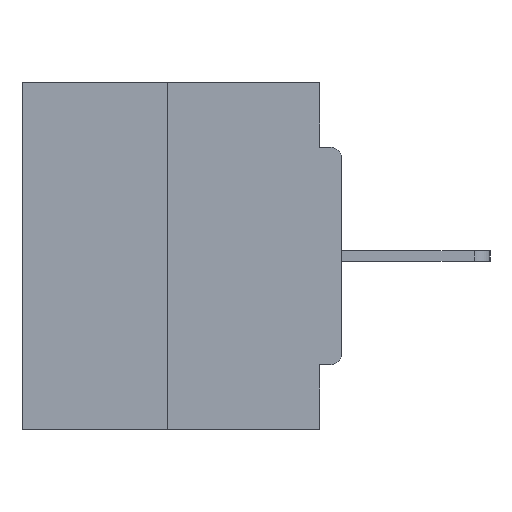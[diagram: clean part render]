
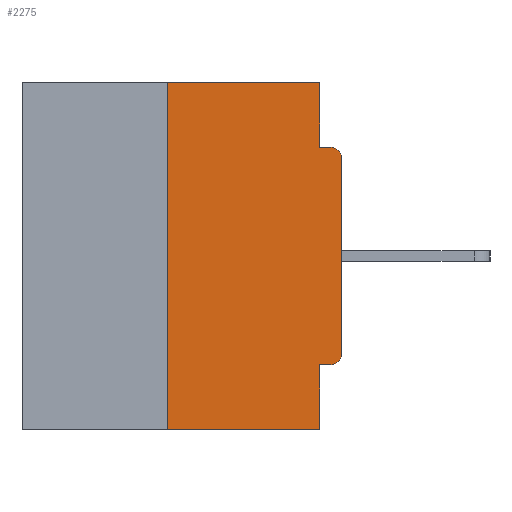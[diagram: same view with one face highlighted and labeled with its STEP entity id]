
A CAD part, left-side view. The second image highlights one B-rep face of the part: STEP entity #2275.
In plain terms, the highlighted planar face has unit normal (-1, 0, 0).
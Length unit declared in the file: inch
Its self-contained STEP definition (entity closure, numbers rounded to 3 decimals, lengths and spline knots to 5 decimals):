
#104 = VECTOR ( 'NONE', #35203, 39.37008 ) ;
#151 = DIRECTION ( 'NONE',  ( 0., 0., -1. ) ) ;
#717 = CARTESIAN_POINT ( 'NONE',  ( 0., 0.031, -0.5 ) ) ;
#1265 = VECTOR ( 'NONE', #12750, 39.37008 ) ;
#1511 = VECTOR ( 'NONE', #16951, 39.37008 ) ;
#1532 = CIRCLE ( 'NONE', #19184, 0.015 ) ;
#1809 = EDGE_CURVE ( 'NONE', #23077, #18736, #36582, .T. ) ;
#2156 = EDGE_CURVE ( 'NONE', #33586, #13961, #5020, .T. ) ;
#2213 = VERTEX_POINT ( 'NONE', #11790 ) ;
#2275 = ADVANCED_FACE ( 'NONE', ( #6070 ), #9224, .F. ) ;
#2962 = DIRECTION ( 'NONE',  ( 0., -1., 0. ) ) ;
#3722 = CARTESIAN_POINT ( 'NONE',  ( 0., 0.015, -0.1085 ) ) ;
#4447 = CARTESIAN_POINT ( 'NONE',  ( 0., 0.031, -0.0935 ) ) ;
#4736 = AXIS2_PLACEMENT_3D ( 'NONE', #36538, #33577, #151 ) ;
#5020 = CIRCLE ( 'NONE', #6319, 0.015 ) ;
#5536 = EDGE_CURVE ( 'NONE', #30319, #26756, #10783, .T. ) ;
#5857 = EDGE_CURVE ( 'NONE', #2213, #18736, #27790, .T. ) ;
#6070 = FACE_OUTER_BOUND ( 'NONE', #24114, .T. ) ;
#6159 = ORIENTED_EDGE ( 'NONE', *, *, #27015, .F. ) ;
#6319 = AXIS2_PLACEMENT_3D ( 'NONE', #11196, #11395, #8246 ) ;
#6888 = EDGE_CURVE ( 'NONE', #33586, #2213, #14207, .T. ) ;
#7771 = ORIENTED_EDGE ( 'NONE', *, *, #5536, .F. ) ;
#8246 = DIRECTION ( 'NONE',  ( 0., 0., -1. ) ) ;
#9224 = PLANE ( 'NONE',  #4736 ) ;
#9358 = CARTESIAN_POINT ( 'NONE',  ( 0., 0.25, 0. ) ) ;
#9653 = ORIENTED_EDGE ( 'NONE', *, *, #29714, .F. ) ;
#10783 = LINE ( 'NONE', #19673, #25838 ) ;
#10842 = CARTESIAN_POINT ( 'NONE',  ( 0., 0., -0.4065 ) ) ;
#11078 = CARTESIAN_POINT ( 'NONE',  ( 0., 0., -0.1085 ) ) ;
#11196 = CARTESIAN_POINT ( 'NONE',  ( 0., 0.015, -0.3915 ) ) ;
#11395 = DIRECTION ( 'NONE',  ( -1., 0., 0. ) ) ;
#11790 = CARTESIAN_POINT ( 'NONE',  ( 0., 0.031, -0.4065 ) ) ;
#11830 = CARTESIAN_POINT ( 'NONE',  ( 0., 0.46, -0.5 ) ) ;
#12288 = VERTEX_POINT ( 'NONE', #11078 ) ;
#12436 = CARTESIAN_POINT ( 'NONE',  ( 0., 0.031, 0. ) ) ;
#12750 = DIRECTION ( 'NONE',  ( 0., 0., -1. ) ) ;
#12808 = ORIENTED_EDGE ( 'NONE', *, *, #16484, .T. ) ;
#12988 = VERTEX_POINT ( 'NONE', #36774 ) ;
#13961 = VERTEX_POINT ( 'NONE', #15565 ) ;
#14040 = VECTOR ( 'NONE', #22882, 39.37008 ) ;
#14207 = LINE ( 'NONE', #10842, #104 ) ;
#14860 = CARTESIAN_POINT ( 'NONE',  ( 0., 0.031, -0.5 ) ) ;
#15407 = ORIENTED_EDGE ( 'NONE', *, *, #6888, .F. ) ;
#15550 = DIRECTION ( 'NONE',  ( 0., 0., -1. ) ) ;
#15565 = CARTESIAN_POINT ( 'NONE',  ( 0., 0., -0.3915 ) ) ;
#15746 = DIRECTION ( 'NONE',  ( -1., 0., 0. ) ) ;
#16277 = VECTOR ( 'NONE', #22070, 39.37008 ) ;
#16484 = EDGE_CURVE ( 'NONE', #13961, #12288, #28609, .T. ) ;
#16951 = DIRECTION ( 'NONE',  ( 0., 0., -1. ) ) ;
#18736 = VERTEX_POINT ( 'NONE', #14860 ) ;
#19184 = AXIS2_PLACEMENT_3D ( 'NONE', #3722, #15746, #15550 ) ;
#19673 = CARTESIAN_POINT ( 'NONE',  ( 0., 0.46, 0. ) ) ;
#20131 = VECTOR ( 'NONE', #2962, 39.37008 ) ;
#20845 = CARTESIAN_POINT ( 'NONE',  ( 0., 0.25, 0. ) ) ;
#22037 = EDGE_CURVE ( 'NONE', #23077, #30319, #33722, .T. ) ;
#22070 = DIRECTION ( 'NONE',  ( 0., 0., 1. ) ) ;
#22587 = ORIENTED_EDGE ( 'NONE', *, *, #5857, .F. ) ;
#22882 = DIRECTION ( 'NONE',  ( 0., -1., 0. ) ) ;
#23077 = VERTEX_POINT ( 'NONE', #35119 ) ;
#23995 = VECTOR ( 'NONE', #36300, 39.37008 ) ;
#24114 = EDGE_LOOP ( 'NONE', ( #7771, #37190, #30785, #22587, #15407, #38112, #12808, #30413, #9653, #6159 ) ) ;
#24303 = VERTEX_POINT ( 'NONE', #4447 ) ;
#25829 = LINE ( 'NONE', #35186, #1511 ) ;
#25838 = VECTOR ( 'NONE', #31775, 39.37008 ) ;
#26415 = CARTESIAN_POINT ( 'NONE',  ( 0., 0.015, -0.4065 ) ) ;
#26756 = VERTEX_POINT ( 'NONE', #12436 ) ;
#27015 = EDGE_CURVE ( 'NONE', #26756, #24303, #25829, .T. ) ;
#27790 = LINE ( 'NONE', #717, #1265 ) ;
#28609 = LINE ( 'NONE', #31578, #16277 ) ;
#28819 = LINE ( 'NONE', #32001, #14040 ) ;
#29714 = EDGE_CURVE ( 'NONE', #24303, #12988, #28819, .T. ) ;
#30319 = VERTEX_POINT ( 'NONE', #20845 ) ;
#30413 = ORIENTED_EDGE ( 'NONE', *, *, #31175, .T. ) ;
#30785 = ORIENTED_EDGE ( 'NONE', *, *, #1809, .T. ) ;
#31175 = EDGE_CURVE ( 'NONE', #12288, #12988, #1532, .T. ) ;
#31578 = CARTESIAN_POINT ( 'NONE',  ( 0., 0., 0. ) ) ;
#31775 = DIRECTION ( 'NONE',  ( 0., -1., 0. ) ) ;
#32001 = CARTESIAN_POINT ( 'NONE',  ( 0., 0., -0.0935 ) ) ;
#33577 = DIRECTION ( 'NONE',  ( 1., 0., 0. ) ) ;
#33586 = VERTEX_POINT ( 'NONE', #26415 ) ;
#33722 = LINE ( 'NONE', #9358, #23995 ) ;
#35119 = CARTESIAN_POINT ( 'NONE',  ( 0., 0.25, -0.5 ) ) ;
#35186 = CARTESIAN_POINT ( 'NONE',  ( 0., 0.031, 0. ) ) ;
#35203 = DIRECTION ( 'NONE',  ( 0., 1., 0. ) ) ;
#36300 = DIRECTION ( 'NONE',  ( 0., 0., 1. ) ) ;
#36538 = CARTESIAN_POINT ( 'NONE',  ( 0., 0.46, 0. ) ) ;
#36582 = LINE ( 'NONE', #11830, #20131 ) ;
#36774 = CARTESIAN_POINT ( 'NONE',  ( 0., 0.015, -0.0935 ) ) ;
#37190 = ORIENTED_EDGE ( 'NONE', *, *, #22037, .F. ) ;
#38112 = ORIENTED_EDGE ( 'NONE', *, *, #2156, .T. ) ;
